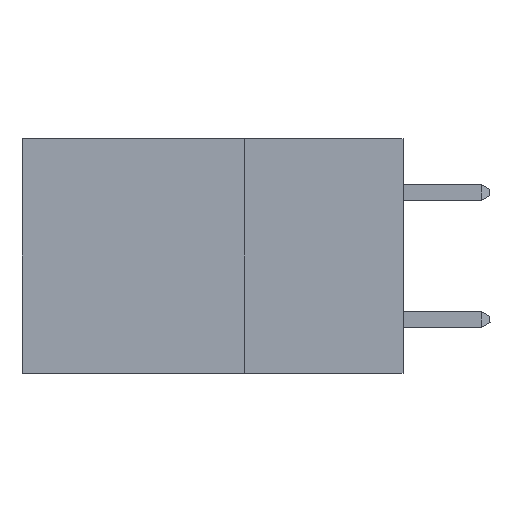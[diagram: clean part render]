
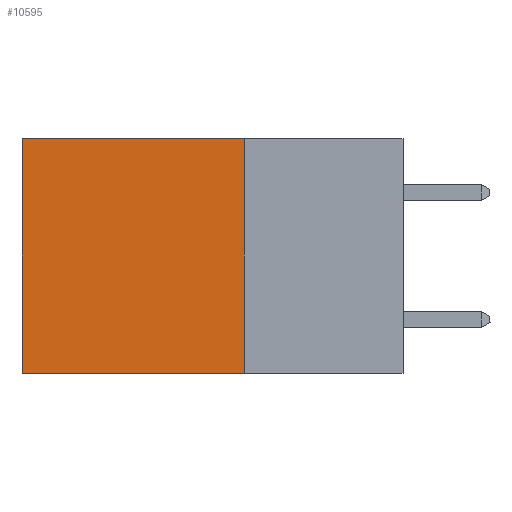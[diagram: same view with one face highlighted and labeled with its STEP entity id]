
A CAD part, left-side view. The second image highlights one B-rep face of the part: STEP entity #10595.
In plain terms, the highlighted planar face has unit normal (-1, 0, 0).
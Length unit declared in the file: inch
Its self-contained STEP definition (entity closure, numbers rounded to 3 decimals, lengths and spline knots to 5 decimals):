
#1199 = CARTESIAN_POINT ( 'NONE',  ( 0.2875, 0.25, 0. ) ) ;
#1282 = VERTEX_POINT ( 'NONE', #12550 ) ;
#2613 = PLANE ( 'NONE',  #8309 ) ;
#3874 = VERTEX_POINT ( 'NONE', #19327 ) ;
#4051 = FACE_OUTER_BOUND ( 'NONE', #13730, .T. ) ;
#4212 = CARTESIAN_POINT ( 'NONE',  ( 0.2875, 0.25, -0.37 ) ) ;
#4813 = DIRECTION ( 'NONE',  ( 0., 1., 0. ) ) ;
#5311 = VECTOR ( 'NONE', #12796, 39.37008 ) ;
#5449 = VECTOR ( 'NONE', #12547, 39.37008 ) ;
#5886 = LINE ( 'NONE', #4212, #18609 ) ;
#7151 = LINE ( 'NONE', #14182, #12418 ) ;
#8126 = EDGE_CURVE ( 'NONE', #1282, #3874, #5886, .T. ) ;
#8182 = LINE ( 'NONE', #19110, #5311 ) ;
#8309 = AXIS2_PLACEMENT_3D ( 'NONE', #1199, #16597, #18190 ) ;
#8425 = CARTESIAN_POINT ( 'NONE',  ( 0.2875, 0.25, 0. ) ) ;
#8924 = ORIENTED_EDGE ( 'NONE', *, *, #8126, .F. ) ;
#9553 = CARTESIAN_POINT ( 'NONE',  ( 0.2875, 0.25, 0. ) ) ;
#10595 = ADVANCED_FACE ( 'NONE', ( #4051 ), #2613, .F. ) ;
#11661 = EDGE_CURVE ( 'NONE', #19865, #19684, #7151, .T. ) ;
#12356 = EDGE_CURVE ( 'NONE', #19865, #1282, #17674, .T. ) ;
#12418 = VECTOR ( 'NONE', #4813, 39.37008 ) ;
#12547 = DIRECTION ( 'NONE',  ( 0., 0., -1. ) ) ;
#12550 = CARTESIAN_POINT ( 'NONE',  ( 0.2875, 0.25, -0.37 ) ) ;
#12796 = DIRECTION ( 'NONE',  ( 0., 0., -1. ) ) ;
#13730 = EDGE_LOOP ( 'NONE', ( #17241, #8924, #15760, #19336 ) ) ;
#14182 = CARTESIAN_POINT ( 'NONE',  ( 0.2875, 0.25, 0. ) ) ;
#15078 = DIRECTION ( 'NONE',  ( 0., 1., 0. ) ) ;
#15760 = ORIENTED_EDGE ( 'NONE', *, *, #12356, .F. ) ;
#16165 = CARTESIAN_POINT ( 'NONE',  ( 0.2875, 0.6, 0. ) ) ;
#16597 = DIRECTION ( 'NONE',  ( 1., 0., 0. ) ) ;
#17241 = ORIENTED_EDGE ( 'NONE', *, *, #18697, .T. ) ;
#17674 = LINE ( 'NONE', #9553, #5449 ) ;
#18190 = DIRECTION ( 'NONE',  ( 0., 0., -1. ) ) ;
#18609 = VECTOR ( 'NONE', #15078, 39.37008 ) ;
#18697 = EDGE_CURVE ( 'NONE', #19684, #3874, #8182, .T. ) ;
#19110 = CARTESIAN_POINT ( 'NONE',  ( 0.2875, 0.6, 0. ) ) ;
#19327 = CARTESIAN_POINT ( 'NONE',  ( 0.2875, 0.6, -0.37 ) ) ;
#19336 = ORIENTED_EDGE ( 'NONE', *, *, #11661, .T. ) ;
#19684 = VERTEX_POINT ( 'NONE', #16165 ) ;
#19865 = VERTEX_POINT ( 'NONE', #8425 ) ;
